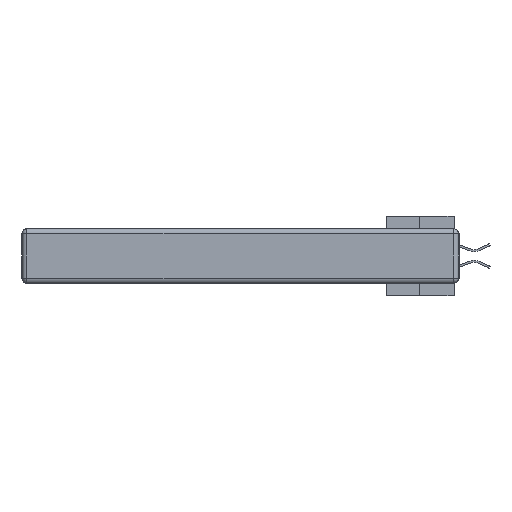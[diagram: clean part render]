
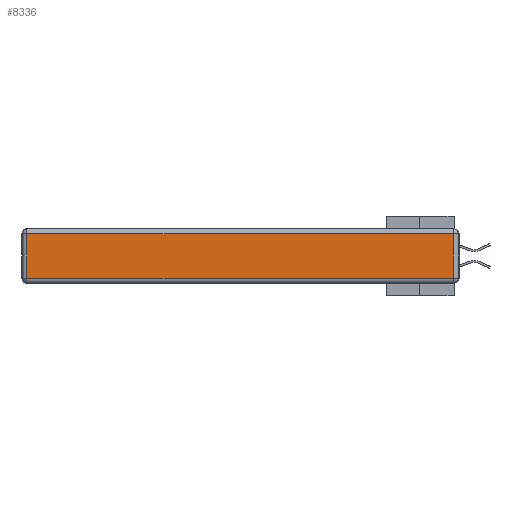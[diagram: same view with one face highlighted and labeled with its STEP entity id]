
A CAD part, left-side view. The second image highlights one B-rep face of the part: STEP entity #8336.
In plain terms, the highlighted planar face has unit normal (-1, 0, 0).
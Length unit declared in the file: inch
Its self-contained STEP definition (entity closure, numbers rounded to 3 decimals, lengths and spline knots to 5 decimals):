
#973 = CARTESIAN_POINT ( 'NONE',  ( 0., 2.72, -0.343 ) ) ;
#2201 = VERTEX_POINT ( 'NONE', #12715 ) ;
#2450 = LINE ( 'NONE', #973, #8519 ) ;
#4725 = VECTOR ( 'NONE', #14024, 39.37008 ) ;
#5588 = CARTESIAN_POINT ( 'NONE',  ( 0., 0.03, -0.313 ) ) ;
#8181 = VECTOR ( 'NONE', #19929, 39.37008 ) ;
#8336 = ADVANCED_FACE ( 'NONE', ( #33095 ), #15686, .T. ) ;
#8519 = VECTOR ( 'NONE', #8831, 39.37008 ) ;
#8731 = CARTESIAN_POINT ( 'NONE',  ( 0., 0., -0.343 ) ) ;
#8831 = DIRECTION ( 'NONE',  ( 0., 0., -1. ) ) ;
#9251 = EDGE_CURVE ( 'NONE', #10018, #31081, #17554, .T. ) ;
#10018 = VERTEX_POINT ( 'NONE', #10362 ) ;
#10362 = CARTESIAN_POINT ( 'NONE',  ( 0., 2.72, -0.313 ) ) ;
#11560 = ORIENTED_EDGE ( 'NONE', *, *, #42340, .T. ) ;
#12269 = DIRECTION ( 'NONE',  ( -1., 0., 0. ) ) ;
#12715 = CARTESIAN_POINT ( 'NONE',  ( 0., 2.72, -0.03 ) ) ;
#14024 = DIRECTION ( 'NONE',  ( 0., 1., 0. ) ) ;
#14133 = LINE ( 'NONE', #20127, #4725 ) ;
#14472 = ORIENTED_EDGE ( 'NONE', *, *, #18068, .T. ) ;
#15686 = PLANE ( 'NONE',  #29995 ) ;
#17554 = LINE ( 'NONE', #30280, #8181 ) ;
#18068 = EDGE_CURVE ( 'NONE', #31081, #32699, #35981, .T. ) ;
#19929 = DIRECTION ( 'NONE',  ( 0., -1., 0. ) ) ;
#20127 = CARTESIAN_POINT ( 'NONE',  ( 0., 2.75, -0.03 ) ) ;
#22440 = EDGE_CURVE ( 'NONE', #2201, #10018, #2450, .T. ) ;
#23068 = DIRECTION ( 'NONE',  ( 0., 0., 1. ) ) ;
#24977 = ORIENTED_EDGE ( 'NONE', *, *, #9251, .T. ) ;
#25947 = ORIENTED_EDGE ( 'NONE', *, *, #22440, .T. ) ;
#27472 = CARTESIAN_POINT ( 'NONE',  ( 0., 0.03, -0.343 ) ) ;
#29995 = AXIS2_PLACEMENT_3D ( 'NONE', #8731, #12269, #23068 ) ;
#30280 = CARTESIAN_POINT ( 'NONE',  ( 0., 0., -0.313 ) ) ;
#31081 = VERTEX_POINT ( 'NONE', #5588 ) ;
#31577 = VECTOR ( 'NONE', #42507, 39.37008 ) ;
#32699 = VERTEX_POINT ( 'NONE', #36211 ) ;
#33095 = FACE_OUTER_BOUND ( 'NONE', #34289, .T. ) ;
#34289 = EDGE_LOOP ( 'NONE', ( #24977, #14472, #11560, #25947 ) ) ;
#35981 = LINE ( 'NONE', #27472, #31577 ) ;
#36211 = CARTESIAN_POINT ( 'NONE',  ( 0., 0.03, -0.03 ) ) ;
#42340 = EDGE_CURVE ( 'NONE', #32699, #2201, #14133, .T. ) ;
#42507 = DIRECTION ( 'NONE',  ( 0., 0., 1. ) ) ;
